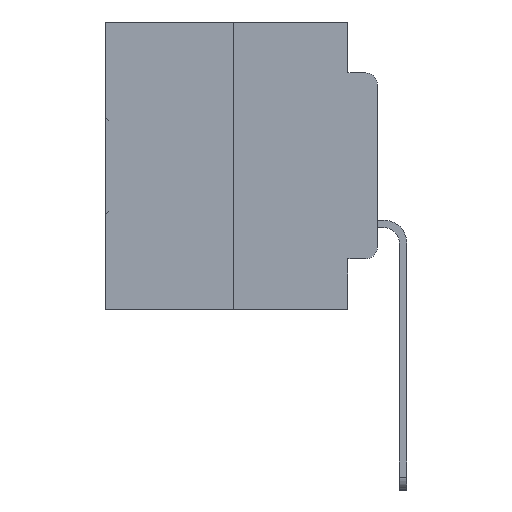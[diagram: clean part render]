
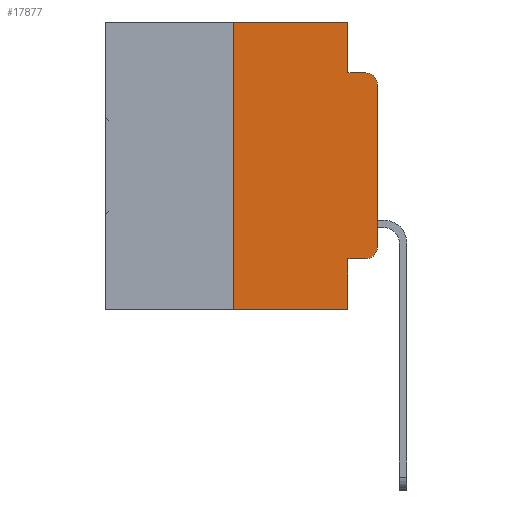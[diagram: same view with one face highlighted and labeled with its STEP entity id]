
A CAD part, left-side view. The second image highlights one B-rep face of the part: STEP entity #17877.
In plain terms, the highlighted planar face has unit normal (-1, 0, 0).
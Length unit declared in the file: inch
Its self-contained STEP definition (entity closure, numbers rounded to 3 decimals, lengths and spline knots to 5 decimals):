
#652 = EDGE_CURVE ( 'NONE', #9172, #31521, #32913, .T. ) ;
#1044 = DIRECTION ( 'NONE',  ( 0., 0., -1. ) ) ;
#1849 = LINE ( 'NONE', #4792, #8364 ) ;
#2140 = VERTEX_POINT ( 'NONE', #9496 ) ;
#2473 = AXIS2_PLACEMENT_3D ( 'NONE', #9230, #26912, #11791 ) ;
#2651 = VERTEX_POINT ( 'NONE', #15267 ) ;
#2680 = EDGE_CURVE ( 'NONE', #26916, #9172, #13355, .T. ) ;
#3307 = ORIENTED_EDGE ( 'NONE', *, *, #19075, .T. ) ;
#3501 = CARTESIAN_POINT ( 'NONE',  ( 0., 0.25, 0. ) ) ;
#3969 = ORIENTED_EDGE ( 'NONE', *, *, #30802, .T. ) ;
#4012 = CARTESIAN_POINT ( 'NONE',  ( 0., 0.051, 0. ) ) ;
#4792 = CARTESIAN_POINT ( 'NONE',  ( 0., 0.051, -0.4115 ) ) ;
#5059 = ORIENTED_EDGE ( 'NONE', *, *, #652, .F. ) ;
#5343 = ORIENTED_EDGE ( 'NONE', *, *, #2680, .F. ) ;
#6193 = CARTESIAN_POINT ( 'NONE',  ( 0., 0., -0.3915 ) ) ;
#6248 = DIRECTION ( 'NONE',  ( 0., 0., 1. ) ) ;
#6646 = CARTESIAN_POINT ( 'NONE',  ( 0., 0.473, 0. ) ) ;
#7314 = ORIENTED_EDGE ( 'NONE', *, *, #15716, .F. ) ;
#7423 = DIRECTION ( 'NONE',  ( 0., -1., 0. ) ) ;
#7885 = CARTESIAN_POINT ( 'NONE',  ( 0., 0.051, -0.0885 ) ) ;
#7893 = DIRECTION ( 'NONE',  ( 0., 0., -1. ) ) ;
#8258 = DIRECTION ( 'NONE',  ( 0., 0., 1. ) ) ;
#8285 = ORIENTED_EDGE ( 'NONE', *, *, #11661, .F. ) ;
#8364 = VECTOR ( 'NONE', #27835, 39.37008 ) ;
#8380 = ORIENTED_EDGE ( 'NONE', *, *, #25245, .T. ) ;
#8617 = ORIENTED_EDGE ( 'NONE', *, *, #16705, .F. ) ;
#9172 = VERTEX_POINT ( 'NONE', #7885 ) ;
#9200 = VECTOR ( 'NONE', #7423, 39.37008 ) ;
#9230 = CARTESIAN_POINT ( 'NONE',  ( 0., 0.02, -0.1085 ) ) ;
#9255 = ORIENTED_EDGE ( 'NONE', *, *, #25287, .T. ) ;
#9444 = ORIENTED_EDGE ( 'NONE', *, *, #26899, .T. ) ;
#9496 = CARTESIAN_POINT ( 'NONE',  ( 0., 0.25, -0.5 ) ) ;
#9791 = DIRECTION ( 'NONE',  ( 1., 0., 0. ) ) ;
#10729 = VERTEX_POINT ( 'NONE', #23773 ) ;
#10850 = VECTOR ( 'NONE', #11806, 39.37008 ) ;
#11661 = EDGE_CURVE ( 'NONE', #2140, #2651, #32225, .T. ) ;
#11791 = DIRECTION ( 'NONE',  ( 0., 0., -1. ) ) ;
#11806 = DIRECTION ( 'NONE',  ( 0., -1., 0. ) ) ;
#12290 = VECTOR ( 'NONE', #6248, 39.37008 ) ;
#12994 = CARTESIAN_POINT ( 'NONE',  ( 0., 0.051, 0. ) ) ;
#13355 = LINE ( 'NONE', #12994, #26027 ) ;
#14193 = FACE_OUTER_BOUND ( 'NONE', #32220, .T. ) ;
#14732 = CARTESIAN_POINT ( 'NONE',  ( 0., 0.051, -0.5 ) ) ;
#15138 = CARTESIAN_POINT ( 'NONE',  ( 0., 0.051, -0.0885 ) ) ;
#15267 = CARTESIAN_POINT ( 'NONE',  ( 0., 0.25, 0. ) ) ;
#15481 = DIRECTION ( 'NONE',  ( 0., 0., -1. ) ) ;
#15716 = EDGE_CURVE ( 'NONE', #2651, #26916, #26627, .T. ) ;
#16633 = VECTOR ( 'NONE', #7893, 39.37008 ) ;
#16705 = EDGE_CURVE ( 'NONE', #31692, #27976, #30785, .T. ) ;
#16940 = DIRECTION ( 'NONE',  ( -1., 0., 0. ) ) ;
#17527 = LINE ( 'NONE', #25289, #9200 ) ;
#17877 = ADVANCED_FACE ( 'NONE', ( #14193 ), #32101, .F. ) ;
#18295 = VERTEX_POINT ( 'NONE', #6193 ) ;
#18907 = VECTOR ( 'NONE', #32626, 39.37008 ) ;
#18997 = VERTEX_POINT ( 'NONE', #25629 ) ;
#19075 = EDGE_CURVE ( 'NONE', #18295, #18997, #33406, .T. ) ;
#21141 = CIRCLE ( 'NONE', #2473, 0.02 ) ;
#22088 = CARTESIAN_POINT ( 'NONE',  ( 0., 0.02, -0.0885 ) ) ;
#22475 = CIRCLE ( 'NONE', #27503, 0.02 ) ;
#23464 = AXIS2_PLACEMENT_3D ( 'NONE', #29777, #9791, #27418 ) ;
#23773 = CARTESIAN_POINT ( 'NONE',  ( 0., 0.02, -0.4115 ) ) ;
#25245 = EDGE_CURVE ( 'NONE', #2140, #27976, #17527, .T. ) ;
#25287 = EDGE_CURVE ( 'NONE', #31692, #10729, #1849, .T. ) ;
#25289 = CARTESIAN_POINT ( 'NONE',  ( 0., 0.473, -0.5 ) ) ;
#25629 = CARTESIAN_POINT ( 'NONE',  ( 0., 0., -0.1085 ) ) ;
#26027 = VECTOR ( 'NONE', #15481, 39.37008 ) ;
#26627 = LINE ( 'NONE', #6646, #10850 ) ;
#26899 = EDGE_CURVE ( 'NONE', #10729, #18295, #22475, .T. ) ;
#26912 = DIRECTION ( 'NONE',  ( -1., 0., 0. ) ) ;
#26914 = VECTOR ( 'NONE', #8258, 39.37008 ) ;
#26916 = VERTEX_POINT ( 'NONE', #4012 ) ;
#27418 = DIRECTION ( 'NONE',  ( 0., 0., -1. ) ) ;
#27503 = AXIS2_PLACEMENT_3D ( 'NONE', #31904, #16940, #1044 ) ;
#27835 = DIRECTION ( 'NONE',  ( 0., -1., 0. ) ) ;
#27976 = VERTEX_POINT ( 'NONE', #14732 ) ;
#29777 = CARTESIAN_POINT ( 'NONE',  ( 0., 0.473, 0. ) ) ;
#30640 = CARTESIAN_POINT ( 'NONE',  ( 0., 0.051, 0. ) ) ;
#30785 = LINE ( 'NONE', #30640, #16633 ) ;
#30802 = EDGE_CURVE ( 'NONE', #18997, #31521, #21141, .T. ) ;
#30851 = CARTESIAN_POINT ( 'NONE',  ( 0., 0., 0. ) ) ;
#31521 = VERTEX_POINT ( 'NONE', #22088 ) ;
#31692 = VERTEX_POINT ( 'NONE', #32527 ) ;
#31904 = CARTESIAN_POINT ( 'NONE',  ( 0., 0.02, -0.3915 ) ) ;
#32101 = PLANE ( 'NONE',  #23464 ) ;
#32220 = EDGE_LOOP ( 'NONE', ( #3307, #3969, #5059, #5343, #7314, #8285, #8380, #8617, #9255, #9444 ) ) ;
#32225 = LINE ( 'NONE', #3501, #12290 ) ;
#32527 = CARTESIAN_POINT ( 'NONE',  ( 0., 0.051, -0.4115 ) ) ;
#32626 = DIRECTION ( 'NONE',  ( 0., -1., 0. ) ) ;
#32913 = LINE ( 'NONE', #15138, #18907 ) ;
#33406 = LINE ( 'NONE', #30851, #26914 ) ;
